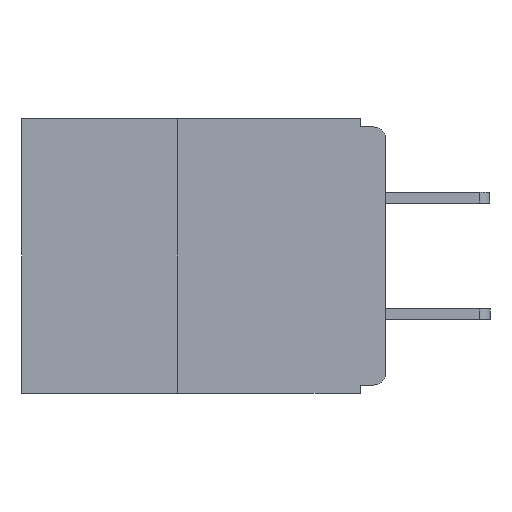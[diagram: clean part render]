
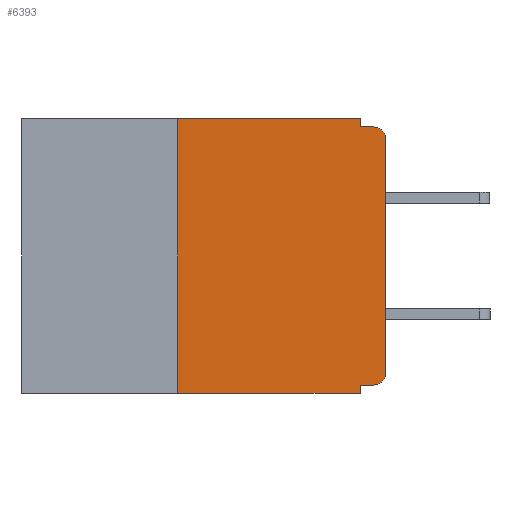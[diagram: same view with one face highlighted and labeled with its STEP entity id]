
A CAD part, left-side view. The second image highlights one B-rep face of the part: STEP entity #6393.
In plain terms, the highlighted planar face has unit normal (-1, 0, 0).
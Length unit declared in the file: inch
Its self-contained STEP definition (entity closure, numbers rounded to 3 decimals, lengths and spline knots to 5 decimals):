
#1151 = DIRECTION ( 'NONE',  ( 0., 0., -1. ) ) ;
#1481 = DIRECTION ( 'NONE',  ( 0., 0., -1. ) ) ;
#2173 = EDGE_CURVE ( 'NONE', #9621, #10868, #4893, .T. ) ;
#2306 = LINE ( 'NONE', #28036, #21592 ) ;
#2742 = CARTESIAN_POINT ( 'NONE',  ( 0., 0., -0.305 ) ) ;
#2825 = DIRECTION ( 'NONE',  ( 0., 0., -1. ) ) ;
#3155 = ORIENTED_EDGE ( 'NONE', *, *, #8076, .F. ) ;
#3544 = ORIENTED_EDGE ( 'NONE', *, *, #2173, .F. ) ;
#3882 = LINE ( 'NONE', #10566, #16400 ) ;
#3948 = VERTEX_POINT ( 'NONE', #2742 ) ;
#4040 = CARTESIAN_POINT ( 'NONE',  ( 0., 0.015, -0.01 ) ) ;
#4230 = FACE_OUTER_BOUND ( 'NONE', #4591, .T. ) ;
#4591 = EDGE_LOOP ( 'NONE', ( #14893, #30555, #15277, #3544, #18426, #20825, #15686, #3155, #25209, #7545 ) ) ;
#4893 = LINE ( 'NONE', #7220, #30743 ) ;
#5357 = EDGE_CURVE ( 'NONE', #20767, #9616, #2306, .T. ) ;
#6393 = ADVANCED_FACE ( 'NONE', ( #4230 ), #25372, .F. ) ;
#7220 = CARTESIAN_POINT ( 'NONE',  ( 0., 0.031, 0. ) ) ;
#7469 = VERTEX_POINT ( 'NONE', #26951 ) ;
#7545 = ORIENTED_EDGE ( 'NONE', *, *, #8117, .T. ) ;
#7832 = EDGE_CURVE ( 'NONE', #10868, #11093, #25459, .T. ) ;
#8076 = EDGE_CURVE ( 'NONE', #14354, #8598, #16725, .T. ) ;
#8117 = EDGE_CURVE ( 'NONE', #27462, #3948, #9328, .T. ) ;
#8134 = DIRECTION ( 'NONE',  ( 0., 0., -1. ) ) ;
#8143 = CARTESIAN_POINT ( 'NONE',  ( 0., 0.031, -0.01 ) ) ;
#8186 = DIRECTION ( 'NONE',  ( 0., -1., 0. ) ) ;
#8598 = VERTEX_POINT ( 'NONE', #13810 ) ;
#9248 = DIRECTION ( 'NONE',  ( -1., 0., 0. ) ) ;
#9328 = CIRCLE ( 'NONE', #29272, 0.015 ) ;
#9616 = VERTEX_POINT ( 'NONE', #23019 ) ;
#9621 = VERTEX_POINT ( 'NONE', #30498 ) ;
#10096 = VECTOR ( 'NONE', #1481, 39.37008 ) ;
#10566 = CARTESIAN_POINT ( 'NONE',  ( 0., 0.437, -0.33 ) ) ;
#10679 = CARTESIAN_POINT ( 'NONE',  ( 0., 0., -0.01 ) ) ;
#10868 = VERTEX_POINT ( 'NONE', #8143 ) ;
#11093 = VERTEX_POINT ( 'NONE', #4040 ) ;
#11598 = EDGE_CURVE ( 'NONE', #27462, #14354, #22077, .T. ) ;
#13186 = CARTESIAN_POINT ( 'NONE',  ( 0., 0.25, -0.33 ) ) ;
#13317 = EDGE_CURVE ( 'NONE', #20767, #8598, #3882, .T. ) ;
#13810 = CARTESIAN_POINT ( 'NONE',  ( 0., 0.031, -0.33 ) ) ;
#14354 = VERTEX_POINT ( 'NONE', #27391 ) ;
#14893 = ORIENTED_EDGE ( 'NONE', *, *, #31830, .T. ) ;
#15277 = ORIENTED_EDGE ( 'NONE', *, *, #7832, .F. ) ;
#15686 = ORIENTED_EDGE ( 'NONE', *, *, #13317, .T. ) ;
#15766 = VECTOR ( 'NONE', #19000, 39.37008 ) ;
#16218 = DIRECTION ( 'NONE',  ( -1., 0., 0. ) ) ;
#16400 = VECTOR ( 'NONE', #30575, 39.37008 ) ;
#16472 = CARTESIAN_POINT ( 'NONE',  ( 0., 0., 0. ) ) ;
#16555 = LINE ( 'NONE', #16472, #15766 ) ;
#16725 = LINE ( 'NONE', #29074, #10096 ) ;
#17833 = DIRECTION ( 'NONE',  ( 1., 0., 0. ) ) ;
#18050 = EDGE_CURVE ( 'NONE', #9616, #9621, #32152, .T. ) ;
#18426 = ORIENTED_EDGE ( 'NONE', *, *, #18050, .F. ) ;
#18700 = CIRCLE ( 'NONE', #19912, 0.015 ) ;
#19000 = DIRECTION ( 'NONE',  ( 0., 0., 1. ) ) ;
#19912 = AXIS2_PLACEMENT_3D ( 'NONE', #31227, #16218, #1151 ) ;
#20767 = VERTEX_POINT ( 'NONE', #13186 ) ;
#20825 = ORIENTED_EDGE ( 'NONE', *, *, #5357, .F. ) ;
#21296 = VECTOR ( 'NONE', #23895, 39.37008 ) ;
#21353 = CARTESIAN_POINT ( 'NONE',  ( 0., 0., -0.32 ) ) ;
#21592 = VECTOR ( 'NONE', #30492, 39.37008 ) ;
#21912 = AXIS2_PLACEMENT_3D ( 'NONE', #30316, #17833, #2825 ) ;
#22077 = LINE ( 'NONE', #21353, #21296 ) ;
#23019 = CARTESIAN_POINT ( 'NONE',  ( 0., 0.25, 0. ) ) ;
#23120 = DIRECTION ( 'NONE',  ( 0., -1., 0. ) ) ;
#23895 = DIRECTION ( 'NONE',  ( 0., 1., 0. ) ) ;
#24299 = CARTESIAN_POINT ( 'NONE',  ( 0., 0.015, -0.305 ) ) ;
#24685 = VECTOR ( 'NONE', #8186, 39.37008 ) ;
#25180 = CARTESIAN_POINT ( 'NONE',  ( 0., 0.015, -0.32 ) ) ;
#25209 = ORIENTED_EDGE ( 'NONE', *, *, #11598, .F. ) ;
#25372 = PLANE ( 'NONE',  #21912 ) ;
#25459 = LINE ( 'NONE', #10679, #24685 ) ;
#25612 = VECTOR ( 'NONE', #23120, 39.37008 ) ;
#26801 = DIRECTION ( 'NONE',  ( 0., 0., -1. ) ) ;
#26951 = CARTESIAN_POINT ( 'NONE',  ( 0., 0., -0.025 ) ) ;
#27391 = CARTESIAN_POINT ( 'NONE',  ( 0., 0.031, -0.32 ) ) ;
#27462 = VERTEX_POINT ( 'NONE', #25180 ) ;
#28036 = CARTESIAN_POINT ( 'NONE',  ( 0., 0.25, -0.33 ) ) ;
#29074 = CARTESIAN_POINT ( 'NONE',  ( 0., 0.031, -0.33 ) ) ;
#29272 = AXIS2_PLACEMENT_3D ( 'NONE', #24299, #9248, #26801 ) ;
#30316 = CARTESIAN_POINT ( 'NONE',  ( 0., 0.437, 0. ) ) ;
#30492 = DIRECTION ( 'NONE',  ( 0., 0., 1. ) ) ;
#30498 = CARTESIAN_POINT ( 'NONE',  ( 0., 0.031, 0. ) ) ;
#30555 = ORIENTED_EDGE ( 'NONE', *, *, #30558, .T. ) ;
#30558 = EDGE_CURVE ( 'NONE', #7469, #11093, #18700, .T. ) ;
#30575 = DIRECTION ( 'NONE',  ( 0., -1., 0. ) ) ;
#30601 = CARTESIAN_POINT ( 'NONE',  ( 0., 0.437, 0. ) ) ;
#30743 = VECTOR ( 'NONE', #8134, 39.37008 ) ;
#31227 = CARTESIAN_POINT ( 'NONE',  ( 0., 0.015, -0.025 ) ) ;
#31830 = EDGE_CURVE ( 'NONE', #3948, #7469, #16555, .T. ) ;
#32152 = LINE ( 'NONE', #30601, #25612 ) ;
